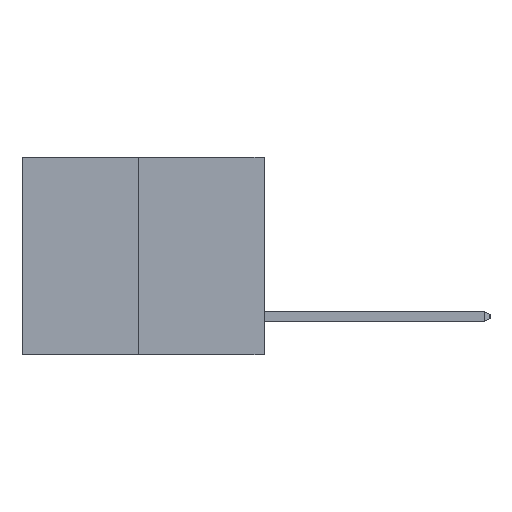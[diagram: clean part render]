
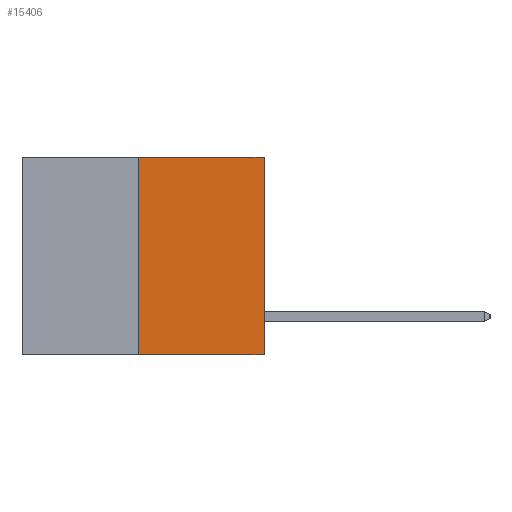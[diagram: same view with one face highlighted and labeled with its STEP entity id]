
A CAD part, left-side view. The second image highlights one B-rep face of the part: STEP entity #15406.
In plain terms, the highlighted planar face has unit normal (-1, 0, 0).
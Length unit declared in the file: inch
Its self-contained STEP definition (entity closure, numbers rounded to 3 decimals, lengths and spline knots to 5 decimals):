
#649 = EDGE_CURVE ( 'NONE', #7154, #5044, #10787, .T. ) ;
#715 = ORIENTED_EDGE ( 'NONE', *, *, #3882, .T. ) ;
#1282 = ORIENTED_EDGE ( 'NONE', *, *, #649, .F. ) ;
#1874 = EDGE_LOOP ( 'NONE', ( #11938, #715, #11266, #1282 ) ) ;
#2156 = LINE ( 'NONE', #4671, #14188 ) ;
#3441 = VERTEX_POINT ( 'NONE', #14505 ) ;
#3628 = DIRECTION ( 'NONE',  ( 1., 0., 0. ) ) ;
#3792 = CARTESIAN_POINT ( 'NONE',  ( 0., 0.312, 0. ) ) ;
#3825 = FACE_OUTER_BOUND ( 'NONE', #1874, .T. ) ;
#3882 = EDGE_CURVE ( 'NONE', #14433, #3441, #4631, .T. ) ;
#4381 = CARTESIAN_POINT ( 'NONE',  ( 0., 0.6, 0. ) ) ;
#4631 = LINE ( 'NONE', #10385, #12904 ) ;
#4651 = CARTESIAN_POINT ( 'NONE',  ( 0., 0.6, 0. ) ) ;
#4671 = CARTESIAN_POINT ( 'NONE',  ( 0., 0.312, -0.49 ) ) ;
#4752 = DIRECTION ( 'NONE',  ( 0., 0., -1. ) ) ;
#4789 = CARTESIAN_POINT ( 'NONE',  ( 0., 0.312, -0.49 ) ) ;
#5044 = VERTEX_POINT ( 'NONE', #11962 ) ;
#5658 = DIRECTION ( 'NONE',  ( 0., -1., 0. ) ) ;
#6318 = LINE ( 'NONE', #10845, #13070 ) ;
#6946 = AXIS2_PLACEMENT_3D ( 'NONE', #4651, #3628, #4752 ) ;
#7146 = DIRECTION ( 'NONE',  ( 0., 0., 1. ) ) ;
#7154 = VERTEX_POINT ( 'NONE', #3792 ) ;
#9838 = EDGE_CURVE ( 'NONE', #14433, #7154, #2156, .T. ) ;
#10385 = CARTESIAN_POINT ( 'NONE',  ( 0., 0.6, -0.49 ) ) ;
#10787 = LINE ( 'NONE', #4381, #12910 ) ;
#10845 = CARTESIAN_POINT ( 'NONE',  ( 0., 0., 0. ) ) ;
#10986 = PLANE ( 'NONE',  #6946 ) ;
#11004 = DIRECTION ( 'NONE',  ( 0., 0., 1. ) ) ;
#11266 = ORIENTED_EDGE ( 'NONE', *, *, #15691, .T. ) ;
#11938 = ORIENTED_EDGE ( 'NONE', *, *, #9838, .F. ) ;
#11947 = DIRECTION ( 'NONE',  ( 0., -1., 0. ) ) ;
#11962 = CARTESIAN_POINT ( 'NONE',  ( 0., 0., 0. ) ) ;
#12904 = VECTOR ( 'NONE', #5658, 39.37008 ) ;
#12910 = VECTOR ( 'NONE', #11947, 39.37008 ) ;
#13070 = VECTOR ( 'NONE', #11004, 39.37008 ) ;
#14188 = VECTOR ( 'NONE', #7146, 39.37008 ) ;
#14433 = VERTEX_POINT ( 'NONE', #4789 ) ;
#14505 = CARTESIAN_POINT ( 'NONE',  ( 0., 0., -0.49 ) ) ;
#15406 = ADVANCED_FACE ( 'NONE', ( #3825 ), #10986, .F. ) ;
#15691 = EDGE_CURVE ( 'NONE', #3441, #5044, #6318, .T. ) ;
